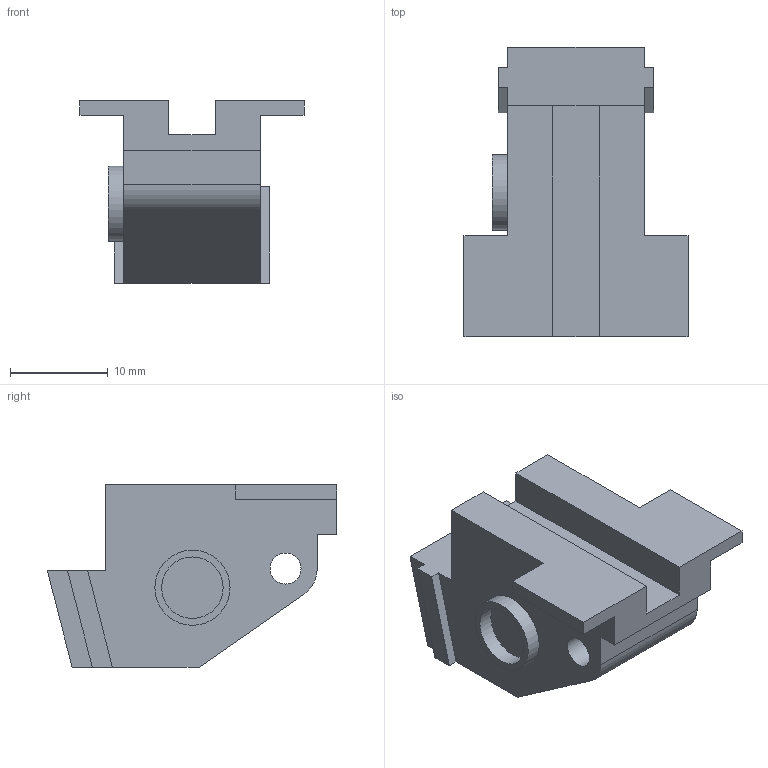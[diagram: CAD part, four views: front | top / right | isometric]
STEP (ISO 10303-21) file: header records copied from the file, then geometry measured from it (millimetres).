
FILE_DESCRIPTION(/* description */ (''),/* implementation_level */ '2;1');
FILE_NAME(/* name */ 'Rear Fire Control Group.step',/* time_stamp */ '2021-03-06T17:01:42-05:00',/* author */ (''),/* organization */ (''),/* preprocessor_version */ 'ST-DEVELOPER v18.1',/* originating_system */ 'Autodesk Translation Framework v9.10.0.1330',/* authorisation */ '');
FILE_SCHEMA (('AUTOMOTIVE_DESIGN { 1 0 10303 214 3 1 1 }'));
Length unit declared in the file: millimetre
Products named in the file (1): Rear Fire Control Group
Bounding box: 22.95 x 29.65 x 18.7 mm (x, y, z)
Volume: 5428.8 mm3; surface area: 2643.4 mm2
Topology: 1 solids, 1 shells, 35 faces, 93 edges, 62 vertices
Faces by surface type: plane 31, cylinder 4
Full cylindrical faces by diameter (mm): 3.18 x1, 6.3 x1, 7.7 x1
Entity records: 1112 total; most frequent: CARTESIAN_POINT 191, ORIENTED_EDGE 186, DIRECTION 173, EDGE_CURVE 93, LINE 85, VECTOR 85, VERTEX_POINT 62, AXIS2_PLACEMENT_3D 44
